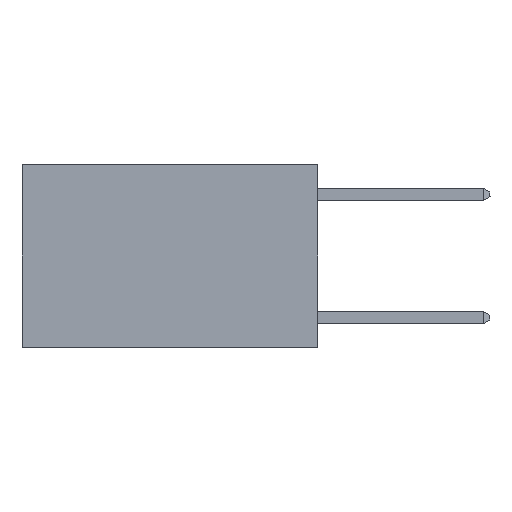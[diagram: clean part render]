
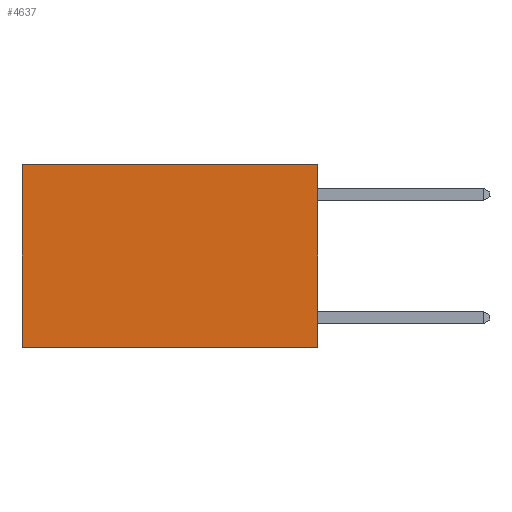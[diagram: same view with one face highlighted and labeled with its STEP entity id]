
A CAD part, left-side view. The second image highlights one B-rep face of the part: STEP entity #4637.
In plain terms, the highlighted planar face has unit normal (-1, 0, 0).
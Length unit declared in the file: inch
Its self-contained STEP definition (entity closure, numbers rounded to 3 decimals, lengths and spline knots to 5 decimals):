
#247 = CARTESIAN_POINT ( 'NONE',  ( 0.2625, 0., 0. ) ) ;
#406 = ORIENTED_EDGE ( 'NONE', *, *, #12426, .F. ) ;
#1001 = CARTESIAN_POINT ( 'NONE',  ( 0.2625, 0., -0.37 ) ) ;
#2446 = PLANE ( 'NONE',  #9113 ) ;
#2525 = CARTESIAN_POINT ( 'NONE',  ( 0.2625, 0., 0. ) ) ;
#2597 = FACE_OUTER_BOUND ( 'NONE', #3322, .T. ) ;
#2956 = ORIENTED_EDGE ( 'NONE', *, *, #9453, .T. ) ;
#3322 = EDGE_LOOP ( 'NONE', ( #2956, #7398, #406, #6695 ) ) ;
#3412 = VERTEX_POINT ( 'NONE', #11675 ) ;
#3451 = DIRECTION ( 'NONE',  ( 0., 0., -1. ) ) ;
#3587 = DIRECTION ( 'NONE',  ( 1., 0., 0. ) ) ;
#3707 = CARTESIAN_POINT ( 'NONE',  ( 0.2625, 0.6, -0.37 ) ) ;
#3968 = VECTOR ( 'NONE', #11096, 39.37008 ) ;
#4107 = LINE ( 'NONE', #8677, #4771 ) ;
#4182 = DIRECTION ( 'NONE',  ( 0., 0., -1. ) ) ;
#4385 = VERTEX_POINT ( 'NONE', #8473 ) ;
#4637 = ADVANCED_FACE ( 'NONE', ( #2597 ), #2446, .F. ) ;
#4771 = VECTOR ( 'NONE', #4182, 39.37008 ) ;
#6695 = ORIENTED_EDGE ( 'NONE', *, *, #9186, .T. ) ;
#6947 = VECTOR ( 'NONE', #11130, 39.37008 ) ;
#7398 = ORIENTED_EDGE ( 'NONE', *, *, #9966, .F. ) ;
#8473 = CARTESIAN_POINT ( 'NONE',  ( 0.2625, 0.6, 0. ) ) ;
#8677 = CARTESIAN_POINT ( 'NONE',  ( 0.2625, 0., 0. ) ) ;
#9113 = AXIS2_PLACEMENT_3D ( 'NONE', #2525, #3587, #3451 ) ;
#9186 = EDGE_CURVE ( 'NONE', #14189, #4385, #12047, .T. ) ;
#9453 = EDGE_CURVE ( 'NONE', #4385, #10141, #10403, .T. ) ;
#9662 = VECTOR ( 'NONE', #11818, 39.37008 ) ;
#9966 = EDGE_CURVE ( 'NONE', #3412, #10141, #13712, .T. ) ;
#9980 = CARTESIAN_POINT ( 'NONE',  ( 0.2625, 0., 0. ) ) ;
#10141 = VERTEX_POINT ( 'NONE', #3707 ) ;
#10403 = LINE ( 'NONE', #10710, #9662 ) ;
#10710 = CARTESIAN_POINT ( 'NONE',  ( 0.2625, 0.6, 0. ) ) ;
#11096 = DIRECTION ( 'NONE',  ( 0., 1., 0. ) ) ;
#11130 = DIRECTION ( 'NONE',  ( 0., 1., 0. ) ) ;
#11675 = CARTESIAN_POINT ( 'NONE',  ( 0.2625, 0., -0.37 ) ) ;
#11818 = DIRECTION ( 'NONE',  ( 0., 0., -1. ) ) ;
#12047 = LINE ( 'NONE', #9980, #3968 ) ;
#12426 = EDGE_CURVE ( 'NONE', #14189, #3412, #4107, .T. ) ;
#13712 = LINE ( 'NONE', #1001, #6947 ) ;
#14189 = VERTEX_POINT ( 'NONE', #247 ) ;
